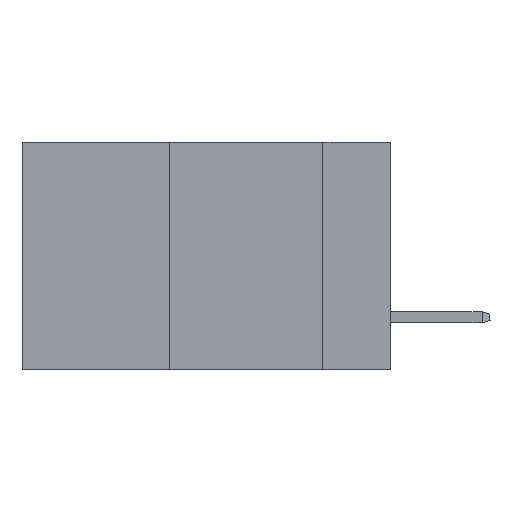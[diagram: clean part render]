
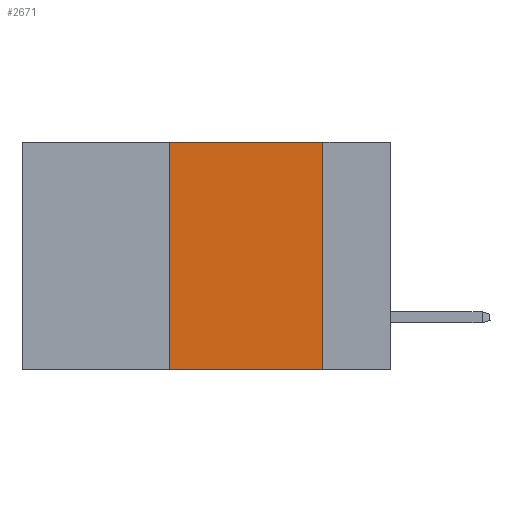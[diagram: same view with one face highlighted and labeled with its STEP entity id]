
A CAD part, left-side view. The second image highlights one B-rep face of the part: STEP entity #2671.
In plain terms, the highlighted planar face has unit normal (-1, 0, 0).
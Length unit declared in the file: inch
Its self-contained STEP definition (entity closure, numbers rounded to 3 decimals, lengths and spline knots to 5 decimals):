
#18 = VERTEX_POINT ( 'NONE', #3148 ) ;
#200 = VERTEX_POINT ( 'NONE', #4738 ) ;
#236 = CARTESIAN_POINT ( 'NONE',  ( 0., 0.11, -0.37 ) ) ;
#1653 = ORIENTED_EDGE ( 'NONE', *, *, #14508, .F. ) ;
#1968 = CARTESIAN_POINT ( 'NONE',  ( 0., 0.11, 0. ) ) ;
#2671 = ADVANCED_FACE ( 'NONE', ( #11193 ), #11154, .F. ) ;
#2674 = VERTEX_POINT ( 'NONE', #3274 ) ;
#2841 = EDGE_CURVE ( 'NONE', #18, #7297, #10660, .T. ) ;
#2849 = EDGE_CURVE ( 'NONE', #2674, #200, #10005, .T. ) ;
#2894 = EDGE_CURVE ( 'NONE', #2674, #7297, #11534, .T. ) ;
#3148 = CARTESIAN_POINT ( 'NONE',  ( 0., 0.11, 0. ) ) ;
#3274 = CARTESIAN_POINT ( 'NONE',  ( 0., 0.36, -0.37 ) ) ;
#4071 = DIRECTION ( 'NONE',  ( 0., -1., 0. ) ) ;
#4110 = DIRECTION ( 'NONE',  ( 0., 0., 1. ) ) ;
#4152 = VECTOR ( 'NONE', #4110, 39.37008 ) ;
#4294 = DIRECTION ( 'NONE',  ( 0., 0., -1. ) ) ;
#4356 = ORIENTED_EDGE ( 'NONE', *, *, #2841, .F. ) ;
#4554 = DIRECTION ( 'NONE',  ( 1., 0., 0. ) ) ;
#4693 = ORIENTED_EDGE ( 'NONE', *, *, #2849, .F. ) ;
#4717 = LINE ( 'NONE', #12688, #7269 ) ;
#4738 = CARTESIAN_POINT ( 'NONE',  ( 0., 0.36, 0. ) ) ;
#4826 = VECTOR ( 'NONE', #4294, 39.37008 ) ;
#6021 = DIRECTION ( 'NONE',  ( 0., -1., 0. ) ) ;
#7113 = EDGE_LOOP ( 'NONE', ( #4356, #1653, #4693, #10536 ) ) ;
#7269 = VECTOR ( 'NONE', #6021, 39.37008 ) ;
#7297 = VERTEX_POINT ( 'NONE', #236 ) ;
#8103 = CARTESIAN_POINT ( 'NONE',  ( 0., 0.6, -0.37 ) ) ;
#8974 = VECTOR ( 'NONE', #4071, 39.37008 ) ;
#10005 = LINE ( 'NONE', #11351, #4152 ) ;
#10536 = ORIENTED_EDGE ( 'NONE', *, *, #2894, .T. ) ;
#10660 = LINE ( 'NONE', #1968, #4826 ) ;
#11154 = PLANE ( 'NONE',  #11269 ) ;
#11193 = FACE_OUTER_BOUND ( 'NONE', #7113, .T. ) ;
#11269 = AXIS2_PLACEMENT_3D ( 'NONE', #12778, #4554, #13525 ) ;
#11351 = CARTESIAN_POINT ( 'NONE',  ( 0., 0.36, 0. ) ) ;
#11534 = LINE ( 'NONE', #8103, #8974 ) ;
#12688 = CARTESIAN_POINT ( 'NONE',  ( 0., 0.6, 0. ) ) ;
#12778 = CARTESIAN_POINT ( 'NONE',  ( 0., 0.6, 0. ) ) ;
#13525 = DIRECTION ( 'NONE',  ( 0., 0., -1. ) ) ;
#14508 = EDGE_CURVE ( 'NONE', #200, #18, #4717, .T. ) ;
